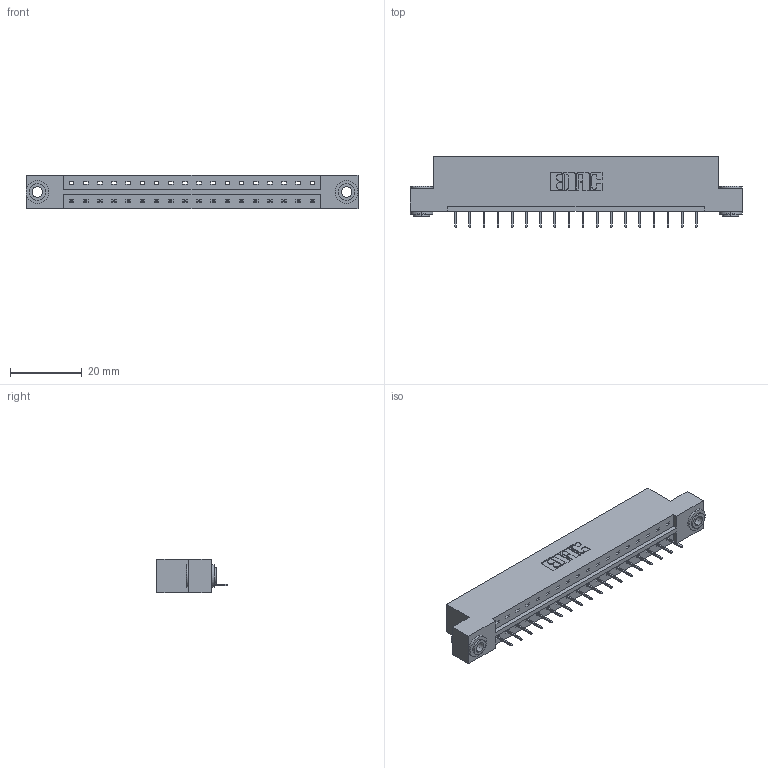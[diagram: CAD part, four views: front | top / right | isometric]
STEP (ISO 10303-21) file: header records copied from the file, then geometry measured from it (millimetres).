
FILE_DESCRIPTION (( 'STEP AP203' ), '1' );
FILE_NAME ('333-018-524-103.STEP', '2019-08-09T13:07:05', ( '' ), ( '' ), 'SwSTEP 2.0', 'SolidWorks 2016', '' );
FILE_SCHEMA (( 'CONFIG_CONTROL_DESIGN' ));
Length unit declared in the file: inch
Products named in the file (4): 345-250-002_345-250-002-102; 345-292-001_345-293-124; 333-018-524-103; 333 Part_Flush - .156 Dia - TH
Assembly tree (21 placements, depth 2):
  333-018-524-103
    333 Part_Flush - .156 Dia - TH
    345-292-001_345-293-124  x18
    345-250-002_345-250-002-102  x2
Bounding box: 92.86 x 19.69 x 9.4 mm (x, y, z)
Volume: 9086.5 mm3; surface area: 9657.5 mm2
Topology: 21 solids, 21 shells, 1268 faces, 3627 edges, 2342 vertices
Faces by surface type: plane 944, cylinder 316, cone 8
Entity records: 14832 total; most frequent: CARTESIAN_POINT 2539, ORIENTED_EDGE 2486, DIRECTION 2225, EDGE_CURVE 1243, VECTOR 1095, LINE 1095, VERTEX_POINT 822, AXIS2_PLACEMENT_3D 565
